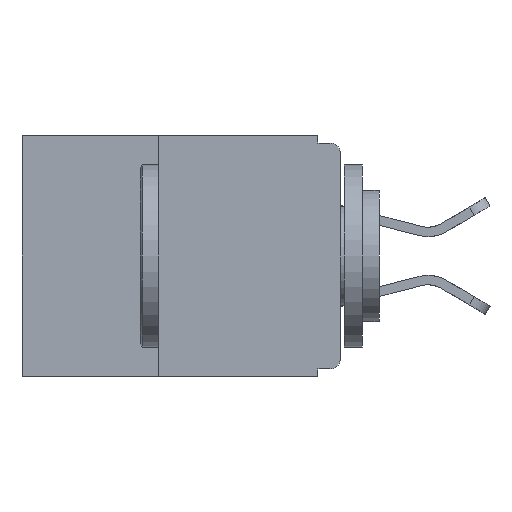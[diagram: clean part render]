
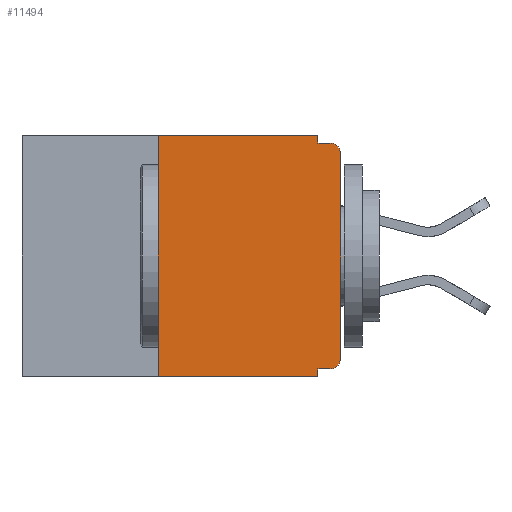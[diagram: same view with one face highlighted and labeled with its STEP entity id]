
A CAD part, left-side view. The second image highlights one B-rep face of the part: STEP entity #11494.
In plain terms, the highlighted planar face has unit normal (-1, 0, 0).
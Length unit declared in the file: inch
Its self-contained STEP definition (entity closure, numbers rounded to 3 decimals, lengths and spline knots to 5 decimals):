
#149 = CARTESIAN_POINT ( 'NONE',  ( 0., 0., -0.305 ) ) ;
#151 = CARTESIAN_POINT ( 'NONE',  ( 0., 0.031, -0.32 ) ) ;
#322 = PLANE ( 'NONE',  #8148 ) ;
#416 = VECTOR ( 'NONE', #6024, 39.37008 ) ;
#746 = VERTEX_POINT ( 'NONE', #9697 ) ;
#876 = ORIENTED_EDGE ( 'NONE', *, *, #12417, .T. ) ;
#1057 = DIRECTION ( 'NONE',  ( 0., -1., 0. ) ) ;
#1201 = ORIENTED_EDGE ( 'NONE', *, *, #4216, .F. ) ;
#1212 = EDGE_CURVE ( 'NONE', #6566, #8917, #5682, .T. ) ;
#1236 = EDGE_CURVE ( 'NONE', #8510, #6529, #12231, .T. ) ;
#1307 = LINE ( 'NONE', #10212, #6085 ) ;
#1380 = VECTOR ( 'NONE', #5948, 39.37008 ) ;
#1397 = ORIENTED_EDGE ( 'NONE', *, *, #10579, .F. ) ;
#1449 = CARTESIAN_POINT ( 'NONE',  ( 0., 0.25, -0.33 ) ) ;
#1699 = VECTOR ( 'NONE', #1057, 39.37008 ) ;
#1718 = ORIENTED_EDGE ( 'NONE', *, *, #3275, .T. ) ;
#1941 = DIRECTION ( 'NONE',  ( 0., 0., -1. ) ) ;
#2051 = ORIENTED_EDGE ( 'NONE', *, *, #1212, .T. ) ;
#2190 = ORIENTED_EDGE ( 'NONE', *, *, #8395, .F. ) ;
#2282 = DIRECTION ( 'NONE',  ( -1., 0., 0. ) ) ;
#2285 = CARTESIAN_POINT ( 'NONE',  ( 0., 0.015, -0.305 ) ) ;
#2411 = VERTEX_POINT ( 'NONE', #7353 ) ;
#2480 = CARTESIAN_POINT ( 'NONE',  ( 0., 0.25, -0.33 ) ) ;
#2804 = VERTEX_POINT ( 'NONE', #7516 ) ;
#3275 = EDGE_CURVE ( 'NONE', #746, #5679, #10610, .T. ) ;
#3368 = LINE ( 'NONE', #5903, #8283 ) ;
#3415 = DIRECTION ( 'NONE',  ( 0., 0., -1. ) ) ;
#3712 = CARTESIAN_POINT ( 'NONE',  ( 0., 0.437, 0. ) ) ;
#4030 = LINE ( 'NONE', #1449, #8876 ) ;
#4118 = LINE ( 'NONE', #8759, #1380 ) ;
#4216 = EDGE_CURVE ( 'NONE', #2411, #7108, #1307, .T. ) ;
#4398 = CARTESIAN_POINT ( 'NONE',  ( 0., 0.437, 0. ) ) ;
#4436 = CARTESIAN_POINT ( 'NONE',  ( 0., 0.031, 0. ) ) ;
#4566 = CARTESIAN_POINT ( 'NONE',  ( 0., 0., 0. ) ) ;
#4727 = ORIENTED_EDGE ( 'NONE', *, *, #9590, .T. ) ;
#5254 = VERTEX_POINT ( 'NONE', #151 ) ;
#5356 = AXIS2_PLACEMENT_3D ( 'NONE', #2285, #2282, #1941 ) ;
#5679 = VERTEX_POINT ( 'NONE', #149 ) ;
#5682 = LINE ( 'NONE', #6326, #9808 ) ;
#5802 = CARTESIAN_POINT ( 'NONE',  ( 0., 0.015, -0.025 ) ) ;
#5855 = ORIENTED_EDGE ( 'NONE', *, *, #11222, .F. ) ;
#5903 = CARTESIAN_POINT ( 'NONE',  ( 0., 0.031, 0. ) ) ;
#5948 = DIRECTION ( 'NONE',  ( 0., 1., 0. ) ) ;
#6024 = DIRECTION ( 'NONE',  ( 0., 0., -1. ) ) ;
#6085 = VECTOR ( 'NONE', #10162, 39.37008 ) ;
#6326 = CARTESIAN_POINT ( 'NONE',  ( 0., 0.437, -0.33 ) ) ;
#6494 = LINE ( 'NONE', #4566, #7089 ) ;
#6529 = VERTEX_POINT ( 'NONE', #4436 ) ;
#6566 = VERTEX_POINT ( 'NONE', #2480 ) ;
#6580 = DIRECTION ( 'NONE',  ( 0., 0., 1. ) ) ;
#6589 = DIRECTION ( 'NONE',  ( 0., -1., 0. ) ) ;
#6797 = DIRECTION ( 'NONE',  ( 0., 0., -1. ) ) ;
#6905 = DIRECTION ( 'NONE',  ( 0., 0., -1. ) ) ;
#7062 = ORIENTED_EDGE ( 'NONE', *, *, #7291, .F. ) ;
#7089 = VECTOR ( 'NONE', #6580, 39.37008 ) ;
#7108 = VERTEX_POINT ( 'NONE', #7212 ) ;
#7212 = CARTESIAN_POINT ( 'NONE',  ( 0., 0.015, -0.01 ) ) ;
#7291 = EDGE_CURVE ( 'NONE', #6566, #8510, #4030, .T. ) ;
#7353 = CARTESIAN_POINT ( 'NONE',  ( 0., 0.031, -0.01 ) ) ;
#7516 = CARTESIAN_POINT ( 'NONE',  ( 0., 0., -0.025 ) ) ;
#7780 = FACE_OUTER_BOUND ( 'NONE', #10558, .T. ) ;
#7931 = LINE ( 'NONE', #12485, #416 ) ;
#8148 = AXIS2_PLACEMENT_3D ( 'NONE', #4398, #9225, #3415 ) ;
#8283 = VECTOR ( 'NONE', #6905, 39.37008 ) ;
#8371 = ORIENTED_EDGE ( 'NONE', *, *, #1236, .F. ) ;
#8395 = EDGE_CURVE ( 'NONE', #6529, #2411, #3368, .T. ) ;
#8510 = VERTEX_POINT ( 'NONE', #9799 ) ;
#8759 = CARTESIAN_POINT ( 'NONE',  ( 0., 0., -0.32 ) ) ;
#8876 = VECTOR ( 'NONE', #9325, 39.37008 ) ;
#8917 = VERTEX_POINT ( 'NONE', #9399 ) ;
#9225 = DIRECTION ( 'NONE',  ( 1., 0., 0. ) ) ;
#9325 = DIRECTION ( 'NONE',  ( 0., 0., 1. ) ) ;
#9399 = CARTESIAN_POINT ( 'NONE',  ( 0., 0.031, -0.33 ) ) ;
#9590 = EDGE_CURVE ( 'NONE', #5679, #2804, #6494, .T. ) ;
#9691 = CIRCLE ( 'NONE', #10504, 0.015 ) ;
#9697 = CARTESIAN_POINT ( 'NONE',  ( 0., 0.015, -0.32 ) ) ;
#9799 = CARTESIAN_POINT ( 'NONE',  ( 0., 0.25, 0. ) ) ;
#9808 = VECTOR ( 'NONE', #6589, 39.37008 ) ;
#10162 = DIRECTION ( 'NONE',  ( 0., -1., 0. ) ) ;
#10212 = CARTESIAN_POINT ( 'NONE',  ( 0., 0., -0.01 ) ) ;
#10504 = AXIS2_PLACEMENT_3D ( 'NONE', #5802, #12298, #6797 ) ;
#10558 = EDGE_LOOP ( 'NONE', ( #4727, #876, #1201, #2190, #8371, #7062, #2051, #5855, #1397, #1718 ) ) ;
#10579 = EDGE_CURVE ( 'NONE', #746, #5254, #4118, .T. ) ;
#10610 = CIRCLE ( 'NONE', #5356, 0.015 ) ;
#11222 = EDGE_CURVE ( 'NONE', #5254, #8917, #7931, .T. ) ;
#11494 = ADVANCED_FACE ( 'NONE', ( #7780 ), #322, .F. ) ;
#12231 = LINE ( 'NONE', #3712, #1699 ) ;
#12298 = DIRECTION ( 'NONE',  ( -1., 0., 0. ) ) ;
#12417 = EDGE_CURVE ( 'NONE', #2804, #7108, #9691, .T. ) ;
#12485 = CARTESIAN_POINT ( 'NONE',  ( 0., 0.031, -0.33 ) ) ;
